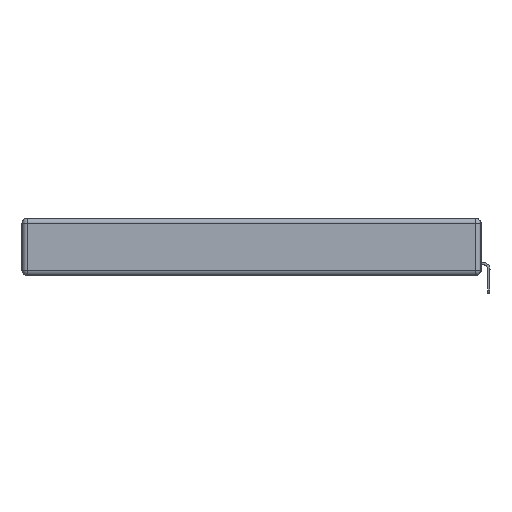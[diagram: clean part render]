
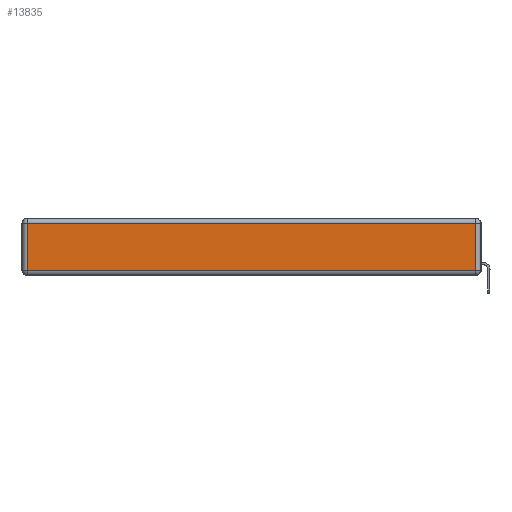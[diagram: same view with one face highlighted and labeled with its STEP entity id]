
A CAD part, left-side view. The second image highlights one B-rep face of the part: STEP entity #13835.
In plain terms, the highlighted planar face has unit normal (-1, 0, 0).
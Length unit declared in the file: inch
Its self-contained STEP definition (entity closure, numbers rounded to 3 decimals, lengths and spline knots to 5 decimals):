
#81 = CARTESIAN_POINT ( 'NONE',  ( 0., 2.72, -0.343 ) ) ;
#554 = PLANE ( 'NONE',  #4160 ) ;
#566 = LINE ( 'NONE', #707, #5955 ) ;
#707 = CARTESIAN_POINT ( 'NONE',  ( 0., 0.03, -0.343 ) ) ;
#1345 = LINE ( 'NONE', #1742, #20186 ) ;
#1357 = VERTEX_POINT ( 'NONE', #9843 ) ;
#1742 = CARTESIAN_POINT ( 'NONE',  ( 0., 2.75, -0.03 ) ) ;
#2427 = DIRECTION ( 'NONE',  ( 0., 0., -1. ) ) ;
#2686 = EDGE_CURVE ( 'NONE', #6532, #6369, #1345, .T. ) ;
#4160 = AXIS2_PLACEMENT_3D ( 'NONE', #12920, #10456, #23081 ) ;
#5955 = VECTOR ( 'NONE', #25698, 39.37008 ) ;
#6369 = VERTEX_POINT ( 'NONE', #7230 ) ;
#6532 = VERTEX_POINT ( 'NONE', #20675 ) ;
#7036 = LINE ( 'NONE', #23783, #20144 ) ;
#7166 = DIRECTION ( 'NONE',  ( 0., -1., 0. ) ) ;
#7230 = CARTESIAN_POINT ( 'NONE',  ( 0., 2.72, -0.03 ) ) ;
#7353 = ORIENTED_EDGE ( 'NONE', *, *, #2686, .T. ) ;
#9756 = VERTEX_POINT ( 'NONE', #17917 ) ;
#9843 = CARTESIAN_POINT ( 'NONE',  ( 0., 2.72, -0.313 ) ) ;
#10456 = DIRECTION ( 'NONE',  ( -1., 0., 0. ) ) ;
#12920 = CARTESIAN_POINT ( 'NONE',  ( 0., 0., -0.343 ) ) ;
#13299 = ORIENTED_EDGE ( 'NONE', *, *, #19473, .T. ) ;
#13835 = ADVANCED_FACE ( 'NONE', ( #17061 ), #554, .T. ) ;
#17061 = FACE_OUTER_BOUND ( 'NONE', #20664, .T. ) ;
#17917 = CARTESIAN_POINT ( 'NONE',  ( 0., 0.03, -0.313 ) ) ;
#17966 = DIRECTION ( 'NONE',  ( 0., 1., 0. ) ) ;
#18982 = ORIENTED_EDGE ( 'NONE', *, *, #25977, .T. ) ;
#19473 = EDGE_CURVE ( 'NONE', #1357, #9756, #7036, .T. ) ;
#20144 = VECTOR ( 'NONE', #7166, 39.37008 ) ;
#20186 = VECTOR ( 'NONE', #17966, 39.37008 ) ;
#20664 = EDGE_LOOP ( 'NONE', ( #13299, #24924, #7353, #18982 ) ) ;
#20675 = CARTESIAN_POINT ( 'NONE',  ( 0., 0.03, -0.03 ) ) ;
#20957 = VECTOR ( 'NONE', #2427, 39.37008 ) ;
#21099 = LINE ( 'NONE', #81, #20957 ) ;
#22875 = EDGE_CURVE ( 'NONE', #9756, #6532, #566, .T. ) ;
#23081 = DIRECTION ( 'NONE',  ( 0., 0., 1. ) ) ;
#23783 = CARTESIAN_POINT ( 'NONE',  ( 0., 0., -0.313 ) ) ;
#24924 = ORIENTED_EDGE ( 'NONE', *, *, #22875, .T. ) ;
#25698 = DIRECTION ( 'NONE',  ( 0., 0., 1. ) ) ;
#25977 = EDGE_CURVE ( 'NONE', #6369, #1357, #21099, .T. ) ;
